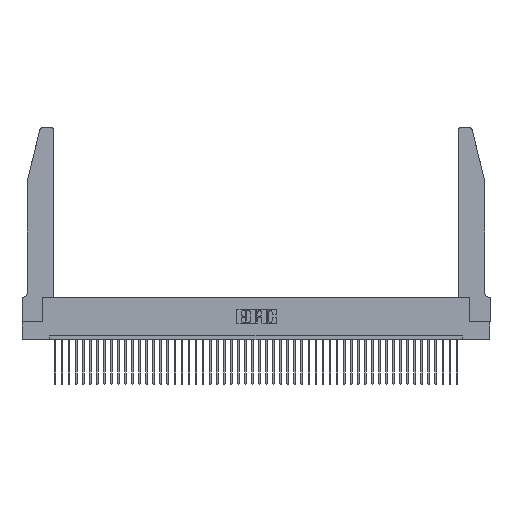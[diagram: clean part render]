
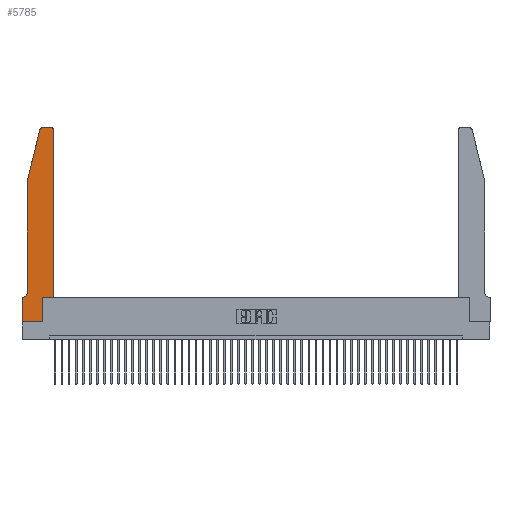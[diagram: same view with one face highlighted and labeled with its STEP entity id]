
A CAD part, top view. The second image highlights one B-rep face of the part: STEP entity #5785.
In plain terms, the highlighted planar face has unit normal (0, 0, 1).
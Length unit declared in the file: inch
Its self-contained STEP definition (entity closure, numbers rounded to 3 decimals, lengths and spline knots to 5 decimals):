
#26 = ORIENTED_EDGE ( 'NONE', *, *, #35409, .T. ) ;
#31 = AXIS2_PLACEMENT_3D ( 'NONE', #38079, #20150, #45081 ) ;
#1023 = DIRECTION ( 'NONE',  ( -1., 0., 0. ) ) ;
#2659 = EDGE_CURVE ( 'NONE', #34417, #4326, #18330, .T. ) ;
#3228 = VECTOR ( 'NONE', #13858, 39.37008 ) ;
#3960 = EDGE_CURVE ( 'NONE', #4326, #5747, #11604, .T. ) ;
#4149 = EDGE_CURVE ( 'NONE', #8803, #34417, #14351, .T. ) ;
#4326 = VERTEX_POINT ( 'NONE', #9212 ) ;
#4668 = DIRECTION ( 'NONE',  ( 0., 0., 1. ) ) ;
#4717 = EDGE_CURVE ( 'NONE', #6814, #11940, #12138, .T. ) ;
#5747 = VERTEX_POINT ( 'NONE', #30333 ) ;
#5785 = ADVANCED_FACE ( 'NONE', ( #11433 ), #29273, .T. ) ;
#5862 = DIRECTION ( 'NONE',  ( -0.239, -0.971, 0. ) ) ;
#6055 = VERTEX_POINT ( 'NONE', #26247 ) ;
#6396 = EDGE_CURVE ( 'NONE', #7221, #6814, #41092, .T. ) ;
#6814 = VERTEX_POINT ( 'NONE', #28874 ) ;
#7221 = VERTEX_POINT ( 'NONE', #26836 ) ;
#7929 = DIRECTION ( 'NONE',  ( 1., 0., 0. ) ) ;
#7984 = EDGE_CURVE ( 'NONE', #6055, #35060, #24683, .T. ) ;
#8193 = VECTOR ( 'NONE', #1023, 39.37008 ) ;
#8733 = ORIENTED_EDGE ( 'NONE', *, *, #6396, .T. ) ;
#8803 = VERTEX_POINT ( 'NONE', #45130 ) ;
#9212 = CARTESIAN_POINT ( 'NONE',  ( 0.25487, 2.72718, 0.37 ) ) ;
#10365 = ORIENTED_EDGE ( 'NONE', *, *, #4717, .T. ) ;
#10591 = CARTESIAN_POINT ( 'NONE',  ( 0.2865, 0.35, 0.37 ) ) ;
#10800 = EDGE_CURVE ( 'NONE', #11940, #34404, #42461, .T. ) ;
#10938 = VERTEX_POINT ( 'NONE', #20459 ) ;
#11018 = VECTOR ( 'NONE', #34316, 39.37008 ) ;
#11032 = DIRECTION ( 'NONE',  ( 1., 0., 0. ) ) ;
#11323 = CARTESIAN_POINT ( 'NONE',  ( 0., 0., 0.37 ) ) ;
#11408 = ORIENTED_EDGE ( 'NONE', *, *, #3960, .T. ) ;
#11433 = FACE_OUTER_BOUND ( 'NONE', #16820, .T. ) ;
#11477 = CARTESIAN_POINT ( 'NONE',  ( 0.4505, 0.35, 0.37 ) ) ;
#11604 = LINE ( 'NONE', #16400, #34556 ) ;
#11940 = VERTEX_POINT ( 'NONE', #11477 ) ;
#12138 = LINE ( 'NONE', #46086, #3228 ) ;
#12139 = LINE ( 'NONE', #37630, #11018 ) ;
#12369 = CARTESIAN_POINT ( 'NONE',  ( 0.4505, 2.72, 0.37 ) ) ;
#13858 = DIRECTION ( 'NONE',  ( 1., 0., 0. ) ) ;
#14200 = DIRECTION ( 'NONE',  ( 0., 0., 1. ) ) ;
#14230 = ORIENTED_EDGE ( 'NONE', *, *, #21344, .T. ) ;
#14351 = LINE ( 'NONE', #22361, #8193 ) ;
#16400 = CARTESIAN_POINT ( 'NONE',  ( 0.0755, 2., 0.37 ) ) ;
#16820 = EDGE_LOOP ( 'NONE', ( #36568, #22065, #11408, #33157, #28127, #14230, #26, #32793, #8733, #10365, #39759, #34501 ) ) ;
#17471 = AXIS2_PLACEMENT_3D ( 'NONE', #39276, #14200, #32300 ) ;
#18085 = CARTESIAN_POINT ( 'NONE',  ( 0., 0., 0.37 ) ) ;
#18330 = CIRCLE ( 'NONE', #17471, 0.03 ) ;
#20150 = DIRECTION ( 'NONE',  ( 0., 0., 1. ) ) ;
#20459 = CARTESIAN_POINT ( 'NONE',  ( 0., 0.35, 0.37 ) ) ;
#21344 = EDGE_CURVE ( 'NONE', #35060, #10938, #12139, .T. ) ;
#21526 = DIRECTION ( 'NONE',  ( 0., 1., 0. ) ) ;
#22050 = CARTESIAN_POINT ( 'NONE',  ( 0., 0.35, 0.37 ) ) ;
#22065 = ORIENTED_EDGE ( 'NONE', *, *, #2659, .T. ) ;
#22361 = CARTESIAN_POINT ( 'NONE',  ( 0.2605, 2.75, 0.37 ) ) ;
#23566 = LINE ( 'NONE', #18085, #29638 ) ;
#24683 = CIRCLE ( 'NONE', #27281, 0.07 ) ;
#25883 = DIRECTION ( 'NONE',  ( 0., 1., 0. ) ) ;
#26247 = CARTESIAN_POINT ( 'NONE',  ( 0.0755, 0.42, 0.37 ) ) ;
#26836 = CARTESIAN_POINT ( 'NONE',  ( 0.2865, 0., 0.37 ) ) ;
#27281 = AXIS2_PLACEMENT_3D ( 'NONE', #43944, #40076, #40551 ) ;
#28127 = ORIENTED_EDGE ( 'NONE', *, *, #7984, .T. ) ;
#28874 = CARTESIAN_POINT ( 'NONE',  ( 0.2865, 0.35, 0.37 ) ) ;
#29273 = PLANE ( 'NONE',  #43127 ) ;
#29638 = VECTOR ( 'NONE', #43431, 39.37008 ) ;
#30333 = CARTESIAN_POINT ( 'NONE',  ( 0.0755, 2., 0.37 ) ) ;
#31120 = CARTESIAN_POINT ( 'NONE',  ( 0.0755, 2., 0.37 ) ) ;
#32152 = EDGE_CURVE ( 'NONE', #34404, #8803, #40135, .T. ) ;
#32300 = DIRECTION ( 'NONE',  ( 1., 0., 0. ) ) ;
#32793 = ORIENTED_EDGE ( 'NONE', *, *, #42802, .T. ) ;
#33098 = CARTESIAN_POINT ( 'NONE',  ( 0.284, 2.75, 0.37 ) ) ;
#33157 = ORIENTED_EDGE ( 'NONE', *, *, #35348, .T. ) ;
#34316 = DIRECTION ( 'NONE',  ( -1., 0., 0. ) ) ;
#34404 = VERTEX_POINT ( 'NONE', #12369 ) ;
#34417 = VERTEX_POINT ( 'NONE', #33098 ) ;
#34501 = ORIENTED_EDGE ( 'NONE', *, *, #32152, .T. ) ;
#34556 = VECTOR ( 'NONE', #5862, 39.37008 ) ;
#35060 = VERTEX_POINT ( 'NONE', #41740 ) ;
#35123 = LINE ( 'NONE', #35466, #41891 ) ;
#35348 = EDGE_CURVE ( 'NONE', #5747, #6055, #35910, .T. ) ;
#35409 = EDGE_CURVE ( 'NONE', #10938, #36740, #23566, .T. ) ;
#35466 = CARTESIAN_POINT ( 'NONE',  ( 0., 0., 0.37 ) ) ;
#35910 = LINE ( 'NONE', #31120, #39329 ) ;
#36568 = ORIENTED_EDGE ( 'NONE', *, *, #4149, .T. ) ;
#36740 = VERTEX_POINT ( 'NONE', #11323 ) ;
#37630 = CARTESIAN_POINT ( 'NONE',  ( 0.0755, 0.35, 0.37 ) ) ;
#38079 = CARTESIAN_POINT ( 'NONE',  ( 0.4205, 2.72, 0.37 ) ) ;
#39016 = DIRECTION ( 'NONE',  ( 0., -1., 0. ) ) ;
#39276 = CARTESIAN_POINT ( 'NONE',  ( 0.284, 2.72, 0.37 ) ) ;
#39329 = VECTOR ( 'NONE', #39016, 39.37008 ) ;
#39759 = ORIENTED_EDGE ( 'NONE', *, *, #10800, .T. ) ;
#40062 = CARTESIAN_POINT ( 'NONE',  ( 0.4505, 0.35, 0.37 ) ) ;
#40076 = DIRECTION ( 'NONE',  ( 0., 0., -1. ) ) ;
#40135 = CIRCLE ( 'NONE', #31, 0.03 ) ;
#40551 = DIRECTION ( 'NONE',  ( -1., 0., 0. ) ) ;
#41092 = LINE ( 'NONE', #10591, #45004 ) ;
#41291 = VECTOR ( 'NONE', #25883, 39.37008 ) ;
#41740 = CARTESIAN_POINT ( 'NONE',  ( 0.0055, 0.35, 0.37 ) ) ;
#41891 = VECTOR ( 'NONE', #11032, 39.37008 ) ;
#42461 = LINE ( 'NONE', #40062, #41291 ) ;
#42802 = EDGE_CURVE ( 'NONE', #36740, #7221, #35123, .T. ) ;
#43127 = AXIS2_PLACEMENT_3D ( 'NONE', #22050, #4668, #7929 ) ;
#43431 = DIRECTION ( 'NONE',  ( 0., -1., 0. ) ) ;
#43944 = CARTESIAN_POINT ( 'NONE',  ( 0.0055, 0.42, 0.37 ) ) ;
#45004 = VECTOR ( 'NONE', #21526, 39.37008 ) ;
#45081 = DIRECTION ( 'NONE',  ( 1., 0., 0. ) ) ;
#45130 = CARTESIAN_POINT ( 'NONE',  ( 0.4205, 2.75, 0.37 ) ) ;
#46086 = CARTESIAN_POINT ( 'NONE',  ( 0.4505, 0.35, 0.37 ) ) ;
